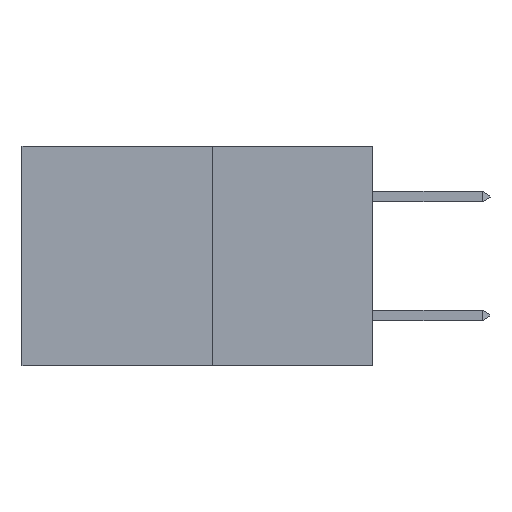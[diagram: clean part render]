
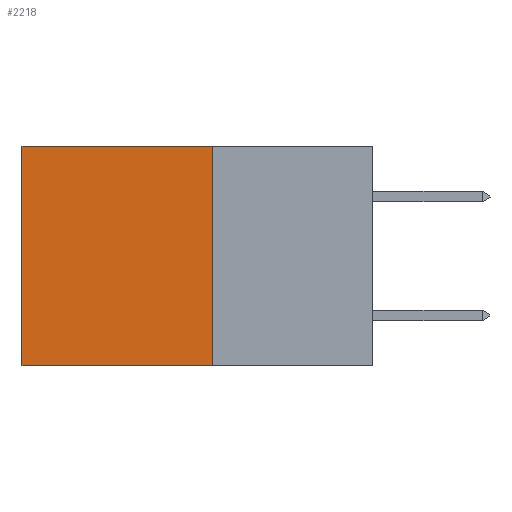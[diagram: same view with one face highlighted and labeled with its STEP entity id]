
A CAD part, left-side view. The second image highlights one B-rep face of the part: STEP entity #2218.
In plain terms, the highlighted planar face has unit normal (-1, 0, 0).
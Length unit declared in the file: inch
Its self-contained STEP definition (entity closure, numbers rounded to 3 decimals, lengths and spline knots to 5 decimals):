
#276 = DIRECTION ( 'NONE',  ( 1., 0., 0. ) ) ;
#297 = VERTEX_POINT ( 'NONE', #3207 ) ;
#502 = PLANE ( 'NONE',  #2394 ) ;
#578 = DIRECTION ( 'NONE',  ( 0., 0., -1. ) ) ;
#852 = EDGE_CURVE ( 'NONE', #2446, #2840, #6259, .T. ) ;
#945 = CARTESIAN_POINT ( 'NONE',  ( 0.277, 0.27, -0.37 ) ) ;
#1199 = FACE_OUTER_BOUND ( 'NONE', #4228, .T. ) ;
#1236 = CARTESIAN_POINT ( 'NONE',  ( 0.277, 0.27, -0.37 ) ) ;
#1363 = CARTESIAN_POINT ( 'NONE',  ( 0.277, 0.27, 0. ) ) ;
#1603 = CARTESIAN_POINT ( 'NONE',  ( 0.277, 0.59, 0. ) ) ;
#1624 = ORIENTED_EDGE ( 'NONE', *, *, #852, .T. ) ;
#1925 = DIRECTION ( 'NONE',  ( 0., 0., -1. ) ) ;
#1928 = VECTOR ( 'NONE', #6194, 39.37008 ) ;
#1941 = CARTESIAN_POINT ( 'NONE',  ( 0.277, 0.59, -0.37 ) ) ;
#2218 = ADVANCED_FACE ( 'NONE', ( #1199 ), #502, .F. ) ;
#2394 = AXIS2_PLACEMENT_3D ( 'NONE', #1236, #276, #578 ) ;
#2446 = VERTEX_POINT ( 'NONE', #1363 ) ;
#2840 = VERTEX_POINT ( 'NONE', #1603 ) ;
#3205 = CARTESIAN_POINT ( 'NONE',  ( 0.277, 0.27, 0. ) ) ;
#3207 = CARTESIAN_POINT ( 'NONE',  ( 0.277, 0.59, -0.37 ) ) ;
#4228 = EDGE_LOOP ( 'NONE', ( #9382, #12222, #9380, #1624 ) ) ;
#4623 = EDGE_CURVE ( 'NONE', #6084, #297, #9858, .T. ) ;
#4773 = VECTOR ( 'NONE', #1925, 39.37008 ) ;
#4876 = EDGE_CURVE ( 'NONE', #2446, #6084, #7436, .T. ) ;
#6084 = VERTEX_POINT ( 'NONE', #10546 ) ;
#6152 = EDGE_CURVE ( 'NONE', #2840, #297, #8650, .T. ) ;
#6194 = DIRECTION ( 'NONE',  ( 0., 1., 0. ) ) ;
#6259 = LINE ( 'NONE', #3205, #8294 ) ;
#6306 = DIRECTION ( 'NONE',  ( 0., 1., 0. ) ) ;
#7436 = LINE ( 'NONE', #945, #4773 ) ;
#8294 = VECTOR ( 'NONE', #6306, 39.37008 ) ;
#8650 = LINE ( 'NONE', #1941, #10822 ) ;
#9380 = ORIENTED_EDGE ( 'NONE', *, *, #4876, .F. ) ;
#9382 = ORIENTED_EDGE ( 'NONE', *, *, #6152, .T. ) ;
#9858 = LINE ( 'NONE', #12177, #1928 ) ;
#10052 = DIRECTION ( 'NONE',  ( 0., 0., -1. ) ) ;
#10546 = CARTESIAN_POINT ( 'NONE',  ( 0.277, 0.27, -0.37 ) ) ;
#10822 = VECTOR ( 'NONE', #10052, 39.37008 ) ;
#12177 = CARTESIAN_POINT ( 'NONE',  ( 0.277, 0.27, -0.37 ) ) ;
#12222 = ORIENTED_EDGE ( 'NONE', *, *, #4623, .F. ) ;
